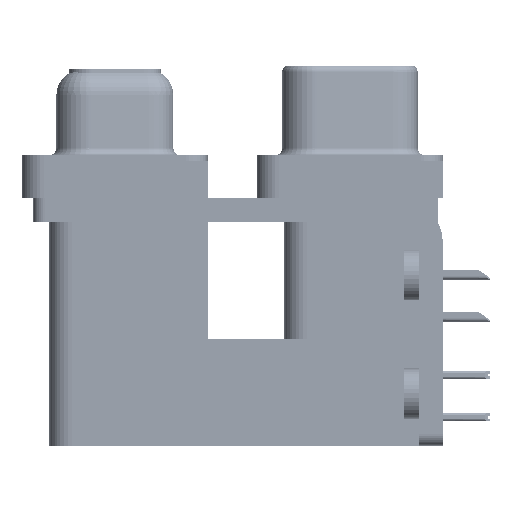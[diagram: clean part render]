
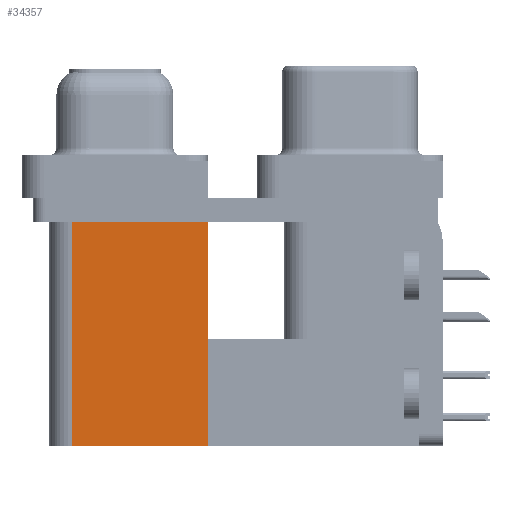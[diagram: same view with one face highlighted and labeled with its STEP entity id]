
A CAD part, left-side view. The second image highlights one B-rep face of the part: STEP entity #34357.
In plain terms, the highlighted planar face has unit normal (-1, 0, 0).
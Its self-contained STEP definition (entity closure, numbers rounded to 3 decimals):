
#1019 = LINE ( 'NONE', #49378, #61047 ) ;
#2875 = EDGE_CURVE ( 'NONE', #55978, #31743, #1019, .T. ) ;
#5650 = DIRECTION ( 'NONE',  ( 0., 1., 0. ) ) ;
#10962 = VECTOR ( 'NONE', #41683, 1000. ) ;
#12428 = AXIS2_PLACEMENT_3D ( 'NONE', #61042, #62094, #23391 ) ;
#16643 = FACE_OUTER_BOUND ( 'NONE', #44863, .T. ) ;
#20854 = ORIENTED_EDGE ( 'NONE', *, *, #44902, .T. ) ;
#21981 = ORIENTED_EDGE ( 'NONE', *, *, #2875, .T. ) ;
#23391 = DIRECTION ( 'NONE',  ( 0., 1., 0. ) ) ;
#24644 = ORIENTED_EDGE ( 'NONE', *, *, #35829, .F. ) ;
#25293 = LINE ( 'NONE', #46985, #45360 ) ;
#26385 = LINE ( 'NONE', #42732, #10962 ) ;
#27421 = VECTOR ( 'NONE', #68164, 1000. ) ;
#28044 = CARTESIAN_POINT ( 'NONE',  ( 3.79, 18.8, -2.5 ) ) ;
#31743 = VERTEX_POINT ( 'NONE', #28044 ) ;
#32807 = CARTESIAN_POINT ( 'NONE',  ( 3.79, 9.6, -19.2 ) ) ;
#34192 = EDGE_CURVE ( 'NONE', #65202, #45390, #25293, .T. ) ;
#34357 = ADVANCED_FACE ( 'NONE', ( #16643 ), #39384, .F. ) ;
#35565 = LINE ( 'NONE', #47272, #27421 ) ;
#35829 = EDGE_CURVE ( 'NONE', #45390, #31743, #35565, .T. ) ;
#39384 = PLANE ( 'NONE',  #12428 ) ;
#41683 = DIRECTION ( 'NONE',  ( 0., 0., 1. ) ) ;
#42732 = CARTESIAN_POINT ( 'NONE',  ( 3.79, 9.6, -19.2 ) ) ;
#44863 = EDGE_LOOP ( 'NONE', ( #21981, #24644, #51687, #20854 ) ) ;
#44902 = EDGE_CURVE ( 'NONE', #65202, #55978, #26385, .T. ) ;
#45360 = VECTOR ( 'NONE', #46307, 1000. ) ;
#45390 = VERTEX_POINT ( 'NONE', #52886 ) ;
#46307 = DIRECTION ( 'NONE',  ( 0., 1., 0. ) ) ;
#46985 = CARTESIAN_POINT ( 'NONE',  ( 3.79, 9.6, -19.2 ) ) ;
#47272 = CARTESIAN_POINT ( 'NONE',  ( 3.79, 18.8, -19.2 ) ) ;
#49378 = CARTESIAN_POINT ( 'NONE',  ( 3.79, 9.6, -2.5 ) ) ;
#51687 = ORIENTED_EDGE ( 'NONE', *, *, #34192, .F. ) ;
#52886 = CARTESIAN_POINT ( 'NONE',  ( 3.79, 18.8, -19.2 ) ) ;
#55324 = CARTESIAN_POINT ( 'NONE',  ( 3.79, 9.6, -2.5 ) ) ;
#55978 = VERTEX_POINT ( 'NONE', #55324 ) ;
#61042 = CARTESIAN_POINT ( 'NONE',  ( 3.79, 9.6, -19.2 ) ) ;
#61047 = VECTOR ( 'NONE', #5650, 1000. ) ;
#62094 = DIRECTION ( 'NONE',  ( 1., 0., 0. ) ) ;
#65202 = VERTEX_POINT ( 'NONE', #32807 ) ;
#68164 = DIRECTION ( 'NONE',  ( 0., 0., 1. ) ) ;
